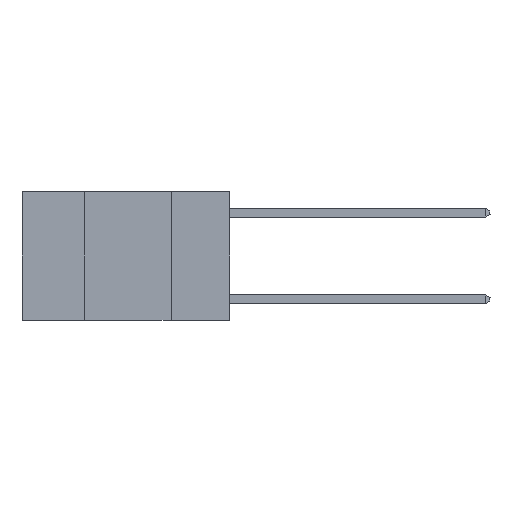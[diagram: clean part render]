
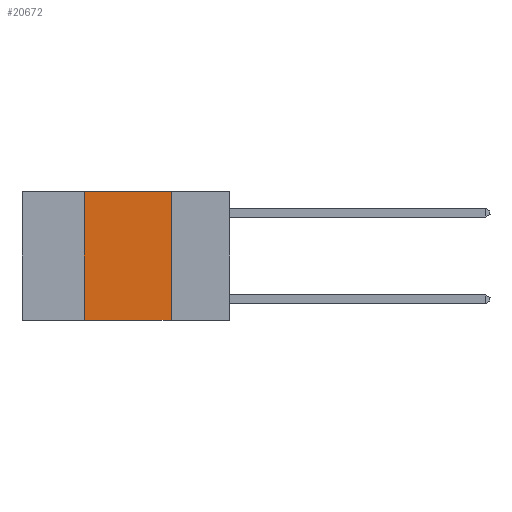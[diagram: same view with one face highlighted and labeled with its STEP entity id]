
A CAD part, left-side view. The second image highlights one B-rep face of the part: STEP entity #20672.
In plain terms, the highlighted planar face has unit normal (-1, 0, 0).
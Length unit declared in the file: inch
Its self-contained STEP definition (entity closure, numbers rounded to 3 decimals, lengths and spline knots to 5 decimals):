
#142 = VECTOR ( 'NONE', #670, 39.37008 ) ;
#670 = DIRECTION ( 'NONE',  ( 0., -1., 0. ) ) ;
#914 = CARTESIAN_POINT ( 'NONE',  ( 0., 0.42, 0. ) ) ;
#1318 = CARTESIAN_POINT ( 'NONE',  ( 0., 0.42, -0.37 ) ) ;
#2269 = LINE ( 'NONE', #19957, #2907 ) ;
#2907 = VECTOR ( 'NONE', #10021, 39.37008 ) ;
#3415 = AXIS2_PLACEMENT_3D ( 'NONE', #23080, #15309, #13241 ) ;
#3693 = CARTESIAN_POINT ( 'NONE',  ( 0., 0.17, 0. ) ) ;
#4010 = LINE ( 'NONE', #23383, #18988 ) ;
#6131 = CARTESIAN_POINT ( 'NONE',  ( 0., 0.6, -0.37 ) ) ;
#6207 = ORIENTED_EDGE ( 'NONE', *, *, #23241, .F. ) ;
#6799 = VERTEX_POINT ( 'NONE', #1318 ) ;
#7639 = PLANE ( 'NONE',  #3415 ) ;
#8193 = ORIENTED_EDGE ( 'NONE', *, *, #8484, .F. ) ;
#8484 = EDGE_CURVE ( 'NONE', #8574, #15717, #2269, .T. ) ;
#8574 = VERTEX_POINT ( 'NONE', #20215 ) ;
#10021 = DIRECTION ( 'NONE',  ( 0., -1., 0. ) ) ;
#10834 = DIRECTION ( 'NONE',  ( 0., 0., 1. ) ) ;
#11231 = VERTEX_POINT ( 'NONE', #21941 ) ;
#13241 = DIRECTION ( 'NONE',  ( 0., 0., -1. ) ) ;
#15309 = DIRECTION ( 'NONE',  ( 1., 0., 0. ) ) ;
#15717 = VERTEX_POINT ( 'NONE', #3693 ) ;
#17099 = FACE_OUTER_BOUND ( 'NONE', #18329, .T. ) ;
#17100 = EDGE_CURVE ( 'NONE', #15717, #11231, #4010, .T. ) ;
#17778 = DIRECTION ( 'NONE',  ( 0., 0., -1. ) ) ;
#18329 = EDGE_LOOP ( 'NONE', ( #21629, #8193, #6207, #22937 ) ) ;
#18984 = EDGE_CURVE ( 'NONE', #6799, #11231, #23610, .T. ) ;
#18988 = VECTOR ( 'NONE', #17778, 39.37008 ) ;
#19957 = CARTESIAN_POINT ( 'NONE',  ( 0., 0.6, 0. ) ) ;
#20199 = VECTOR ( 'NONE', #10834, 39.37008 ) ;
#20215 = CARTESIAN_POINT ( 'NONE',  ( 0., 0.42, 0. ) ) ;
#20672 = ADVANCED_FACE ( 'NONE', ( #17099 ), #7639, .F. ) ;
#21629 = ORIENTED_EDGE ( 'NONE', *, *, #17100, .F. ) ;
#21941 = CARTESIAN_POINT ( 'NONE',  ( 0., 0.17, -0.37 ) ) ;
#22937 = ORIENTED_EDGE ( 'NONE', *, *, #18984, .T. ) ;
#23080 = CARTESIAN_POINT ( 'NONE',  ( 0., 0.6, 0. ) ) ;
#23241 = EDGE_CURVE ( 'NONE', #6799, #8574, #24347, .T. ) ;
#23383 = CARTESIAN_POINT ( 'NONE',  ( 0., 0.17, 0. ) ) ;
#23610 = LINE ( 'NONE', #6131, #142 ) ;
#24347 = LINE ( 'NONE', #914, #20199 ) ;
